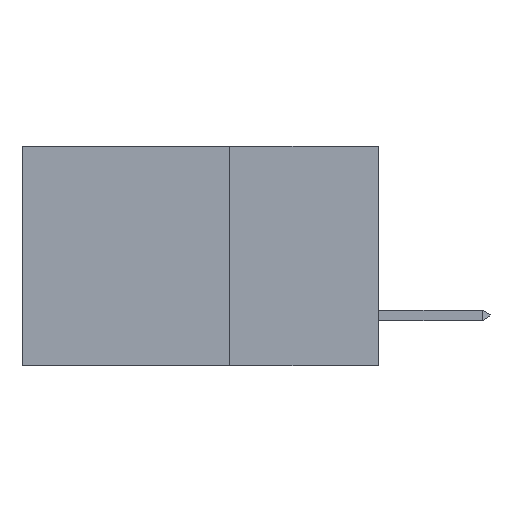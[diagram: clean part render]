
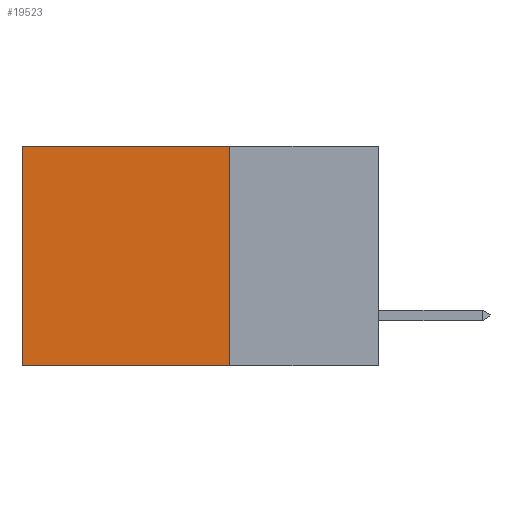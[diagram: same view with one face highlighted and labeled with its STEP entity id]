
A CAD part, left-side view. The second image highlights one B-rep face of the part: STEP entity #19523.
In plain terms, the highlighted planar face has unit normal (-1, 0, 0).
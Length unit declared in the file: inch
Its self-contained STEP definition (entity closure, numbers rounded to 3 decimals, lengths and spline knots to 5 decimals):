
#1130 = CARTESIAN_POINT ( 'NONE',  ( 0.298, 0.25, 0. ) ) ;
#1718 = VECTOR ( 'NONE', #4550, 39.37008 ) ;
#1937 = LINE ( 'NONE', #16691, #13762 ) ;
#2480 = LINE ( 'NONE', #13914, #1718 ) ;
#2912 = DIRECTION ( 'NONE',  ( 0., 1., 0. ) ) ;
#3502 = DIRECTION ( 'NONE',  ( 0., 1., 0. ) ) ;
#4418 = EDGE_LOOP ( 'NONE', ( #25292, #4674, #12902, #24500 ) ) ;
#4550 = DIRECTION ( 'NONE',  ( 0., 0., -1. ) ) ;
#4674 = ORIENTED_EDGE ( 'NONE', *, *, #8723, .F. ) ;
#4964 = DIRECTION ( 'NONE',  ( 0., 0., -1. ) ) ;
#5679 = LINE ( 'NONE', #19978, #11198 ) ;
#5862 = EDGE_CURVE ( 'NONE', #7965, #16368, #2480, .T. ) ;
#5936 = DIRECTION ( 'NONE',  ( 0., 0., -1. ) ) ;
#6816 = FACE_OUTER_BOUND ( 'NONE', #4418, .T. ) ;
#7250 = VERTEX_POINT ( 'NONE', #16523 ) ;
#7321 = CARTESIAN_POINT ( 'NONE',  ( 0.298, 0.6, -0.37 ) ) ;
#7344 = CARTESIAN_POINT ( 'NONE',  ( 0.298, 0.25, 0. ) ) ;
#7965 = VERTEX_POINT ( 'NONE', #7344 ) ;
#8723 = EDGE_CURVE ( 'NONE', #16368, #21607, #5679, .T. ) ;
#9614 = LINE ( 'NONE', #17021, #28486 ) ;
#11198 = VECTOR ( 'NONE', #3502, 39.37008 ) ;
#12312 = AXIS2_PLACEMENT_3D ( 'NONE', #1130, #20019, #5936 ) ;
#12902 = ORIENTED_EDGE ( 'NONE', *, *, #5862, .F. ) ;
#13762 = VECTOR ( 'NONE', #4964, 39.37008 ) ;
#13914 = CARTESIAN_POINT ( 'NONE',  ( 0.298, 0.25, 0. ) ) ;
#15285 = PLANE ( 'NONE',  #12312 ) ;
#16368 = VERTEX_POINT ( 'NONE', #27959 ) ;
#16523 = CARTESIAN_POINT ( 'NONE',  ( 0.298, 0.6, 0. ) ) ;
#16691 = CARTESIAN_POINT ( 'NONE',  ( 0.298, 0.6, 0. ) ) ;
#17021 = CARTESIAN_POINT ( 'NONE',  ( 0.298, 0.25, 0. ) ) ;
#19523 = ADVANCED_FACE ( 'NONE', ( #6816 ), #15285, .F. ) ;
#19921 = EDGE_CURVE ( 'NONE', #7250, #21607, #1937, .T. ) ;
#19978 = CARTESIAN_POINT ( 'NONE',  ( 0.298, 0.25, -0.37 ) ) ;
#20019 = DIRECTION ( 'NONE',  ( 1., 0., 0. ) ) ;
#21607 = VERTEX_POINT ( 'NONE', #7321 ) ;
#22905 = EDGE_CURVE ( 'NONE', #7965, #7250, #9614, .T. ) ;
#24500 = ORIENTED_EDGE ( 'NONE', *, *, #22905, .T. ) ;
#25292 = ORIENTED_EDGE ( 'NONE', *, *, #19921, .T. ) ;
#27959 = CARTESIAN_POINT ( 'NONE',  ( 0.298, 0.25, -0.37 ) ) ;
#28486 = VECTOR ( 'NONE', #2912, 39.37008 ) ;
